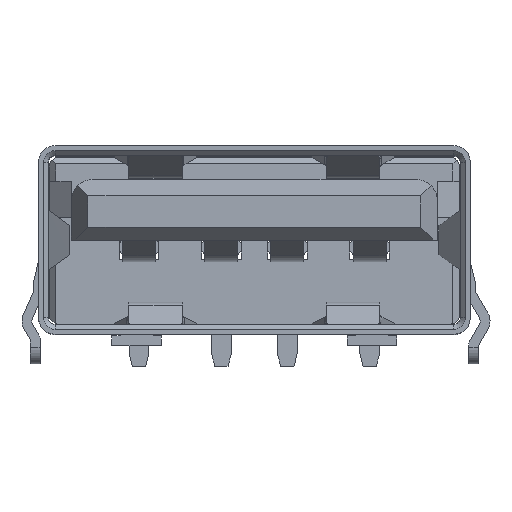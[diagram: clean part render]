
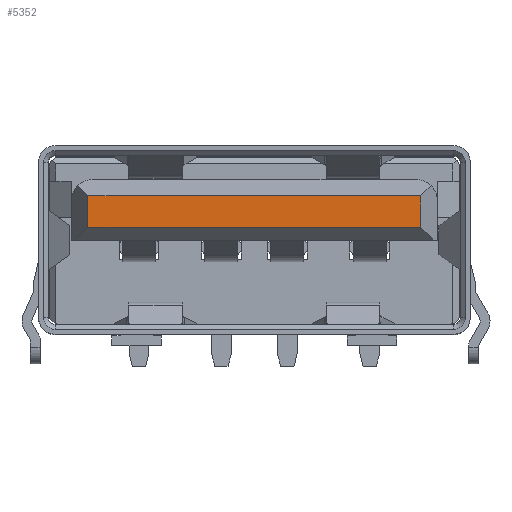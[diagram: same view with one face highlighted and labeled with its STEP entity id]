
A CAD part, top view. The second image highlights one B-rep face of the part: STEP entity #5352.
In plain terms, the highlighted planar face has unit normal (0, 0, 1).
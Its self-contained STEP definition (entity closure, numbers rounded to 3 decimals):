
#81 = CARTESIAN_POINT ( 'NONE',  ( 6.225, -1.67, 8.38 ) ) ;
#899 = ORIENTED_EDGE ( 'NONE', *, *, #15336, .F. ) ;
#1196 = CARTESIAN_POINT ( 'NONE',  ( 6.225, -1.19, 8.38 ) ) ;
#2117 = LINE ( 'NONE', #15468, #5502 ) ;
#2920 = DIRECTION ( 'NONE',  ( 0., -1., 0. ) ) ;
#3065 = VERTEX_POINT ( 'NONE', #17127 ) ;
#4259 = VERTEX_POINT ( 'NONE', #12483 ) ;
#4510 = VECTOR ( 'NONE', #2920, 1000. ) ;
#4658 = VECTOR ( 'NONE', #5958, 1000. ) ;
#5352 = ADVANCED_FACE ( 'NONE', ( #17539 ), #8588, .F. ) ;
#5502 = VECTOR ( 'NONE', #18422, 1000. ) ;
#5958 = DIRECTION ( 'NONE',  ( 1., 0., 0. ) ) ;
#6272 = ORIENTED_EDGE ( 'NONE', *, *, #17554, .F. ) ;
#7038 = DIRECTION ( 'NONE',  ( 1., 0., 0. ) ) ;
#7608 = EDGE_CURVE ( 'NONE', #4259, #18788, #2117, .T. ) ;
#7968 = CARTESIAN_POINT ( 'NONE',  ( 11.275, -2.15, 8.38 ) ) ;
#8588 = PLANE ( 'NONE',  #13504 ) ;
#10081 = LINE ( 'NONE', #1196, #15038 ) ;
#10168 = ORIENTED_EDGE ( 'NONE', *, *, #7608, .T. ) ;
#10429 = CARTESIAN_POINT ( 'NONE',  ( 6.225, -2.15, 8.38 ) ) ;
#10574 = EDGE_LOOP ( 'NONE', ( #899, #10168, #13631, #6272 ) ) ;
#10637 = LINE ( 'NONE', #16157, #4510 ) ;
#11580 = CARTESIAN_POINT ( 'NONE',  ( 1.175, -2.15, 8.38 ) ) ;
#12483 = CARTESIAN_POINT ( 'NONE',  ( 1.175, -1.19, 8.38 ) ) ;
#12946 = EDGE_CURVE ( 'NONE', #18788, #17737, #17838, .T. ) ;
#12964 = DIRECTION ( 'NONE',  ( 0., 0., -1. ) ) ;
#13049 = DIRECTION ( 'NONE',  ( -1., 0., 0. ) ) ;
#13504 = AXIS2_PLACEMENT_3D ( 'NONE', #81, #12964, #13049 ) ;
#13631 = ORIENTED_EDGE ( 'NONE', *, *, #12946, .T. ) ;
#15038 = VECTOR ( 'NONE', #7038, 1000. ) ;
#15336 = EDGE_CURVE ( 'NONE', #4259, #3065, #10081, .T. ) ;
#15468 = CARTESIAN_POINT ( 'NONE',  ( 1.175, -1.704, 8.38 ) ) ;
#16157 = CARTESIAN_POINT ( 'NONE',  ( 11.275, -1.67, 8.38 ) ) ;
#17127 = CARTESIAN_POINT ( 'NONE',  ( 11.275, -1.19, 8.38 ) ) ;
#17539 = FACE_OUTER_BOUND ( 'NONE', #10574, .T. ) ;
#17554 = EDGE_CURVE ( 'NONE', #3065, #17737, #10637, .T. ) ;
#17737 = VERTEX_POINT ( 'NONE', #7968 ) ;
#17838 = LINE ( 'NONE', #10429, #4658 ) ;
#18422 = DIRECTION ( 'NONE',  ( 0., -1., 0. ) ) ;
#18788 = VERTEX_POINT ( 'NONE', #11580 ) ;
